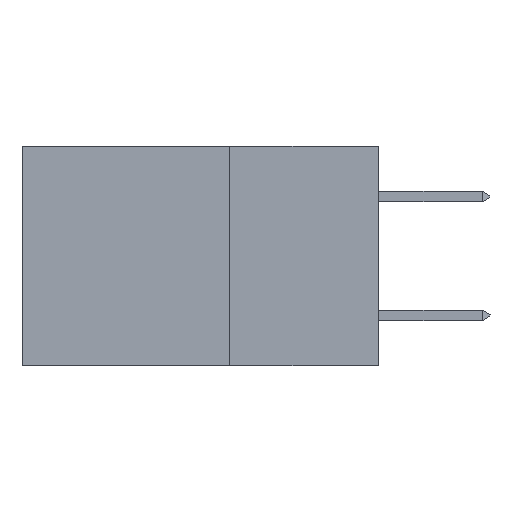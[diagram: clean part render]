
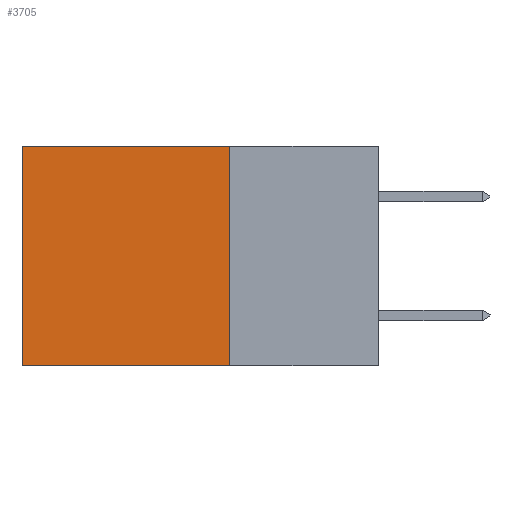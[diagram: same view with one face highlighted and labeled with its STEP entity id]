
A CAD part, left-side view. The second image highlights one B-rep face of the part: STEP entity #3705.
In plain terms, the highlighted planar face has unit normal (-1, 0, 0).
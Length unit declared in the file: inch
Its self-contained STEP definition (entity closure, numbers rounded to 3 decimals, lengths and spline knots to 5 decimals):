
#134 = EDGE_CURVE ( 'NONE', #3447, #3926, #2240, .T. ) ;
#818 = ORIENTED_EDGE ( 'NONE', *, *, #9965, .F. ) ;
#1405 = ORIENTED_EDGE ( 'NONE', *, *, #134, .F. ) ;
#1498 = LINE ( 'NONE', #4073, #8366 ) ;
#1574 = LINE ( 'NONE', #7639, #1873 ) ;
#1873 = VECTOR ( 'NONE', #11813, 39.37008 ) ;
#2127 = CARTESIAN_POINT ( 'NONE',  ( 0.298, 0.25, 0. ) ) ;
#2240 = LINE ( 'NONE', #2127, #7007 ) ;
#2430 = VECTOR ( 'NONE', #8171, 39.37008 ) ;
#3447 = VERTEX_POINT ( 'NONE', #8768 ) ;
#3705 = ADVANCED_FACE ( 'NONE', ( #7002 ), #5288, .F. ) ;
#3926 = VERTEX_POINT ( 'NONE', #10327 ) ;
#4073 = CARTESIAN_POINT ( 'NONE',  ( 0.298, 0.25, -0.37 ) ) ;
#4301 = DIRECTION ( 'NONE',  ( 0., 0., -1. ) ) ;
#4436 = VERTEX_POINT ( 'NONE', #11493 ) ;
#4940 = ORIENTED_EDGE ( 'NONE', *, *, #6639, .T. ) ;
#5288 = PLANE ( 'NONE',  #9968 ) ;
#5769 = CARTESIAN_POINT ( 'NONE',  ( 0.298, 0.6, 0. ) ) ;
#6247 = DIRECTION ( 'NONE',  ( 0., 0., -1. ) ) ;
#6294 = DIRECTION ( 'NONE',  ( 1., 0., 0. ) ) ;
#6518 = ORIENTED_EDGE ( 'NONE', *, *, #13024, .T. ) ;
#6639 = EDGE_CURVE ( 'NONE', #7431, #4436, #12079, .T. ) ;
#7002 = FACE_OUTER_BOUND ( 'NONE', #8893, .T. ) ;
#7007 = VECTOR ( 'NONE', #6247, 39.37008 ) ;
#7431 = VERTEX_POINT ( 'NONE', #5769 ) ;
#7639 = CARTESIAN_POINT ( 'NONE',  ( 0.298, 0.25, 0. ) ) ;
#7817 = DIRECTION ( 'NONE',  ( 0., 1., 0. ) ) ;
#8171 = DIRECTION ( 'NONE',  ( 0., 0., -1. ) ) ;
#8366 = VECTOR ( 'NONE', #7817, 39.37008 ) ;
#8768 = CARTESIAN_POINT ( 'NONE',  ( 0.298, 0.25, 0. ) ) ;
#8893 = EDGE_LOOP ( 'NONE', ( #4940, #818, #1405, #6518 ) ) ;
#9965 = EDGE_CURVE ( 'NONE', #3926, #4436, #1498, .T. ) ;
#9968 = AXIS2_PLACEMENT_3D ( 'NONE', #12507, #6294, #4301 ) ;
#10327 = CARTESIAN_POINT ( 'NONE',  ( 0.298, 0.25, -0.37 ) ) ;
#11446 = CARTESIAN_POINT ( 'NONE',  ( 0.298, 0.6, 0. ) ) ;
#11493 = CARTESIAN_POINT ( 'NONE',  ( 0.298, 0.6, -0.37 ) ) ;
#11813 = DIRECTION ( 'NONE',  ( 0., 1., 0. ) ) ;
#12079 = LINE ( 'NONE', #11446, #2430 ) ;
#12507 = CARTESIAN_POINT ( 'NONE',  ( 0.298, 0.25, 0. ) ) ;
#13024 = EDGE_CURVE ( 'NONE', #3447, #7431, #1574, .T. ) ;
